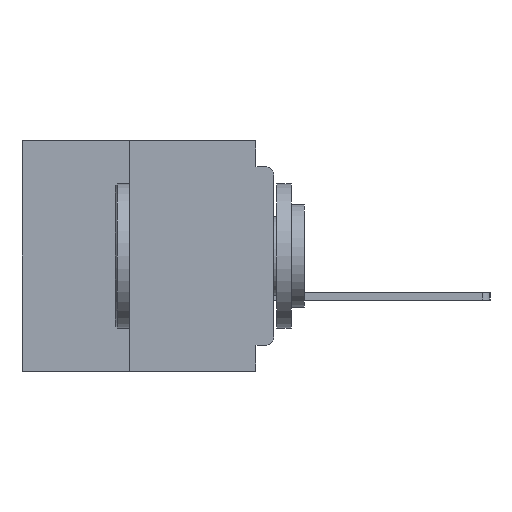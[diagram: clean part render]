
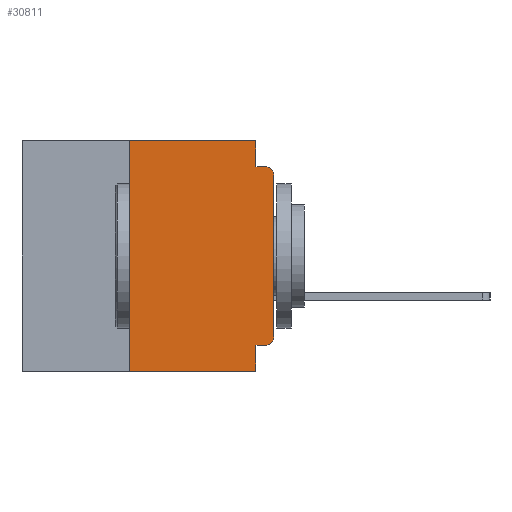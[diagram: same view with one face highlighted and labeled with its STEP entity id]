
A CAD part, left-side view. The second image highlights one B-rep face of the part: STEP entity #30811.
In plain terms, the highlighted planar face has unit normal (-1, 0, 0).
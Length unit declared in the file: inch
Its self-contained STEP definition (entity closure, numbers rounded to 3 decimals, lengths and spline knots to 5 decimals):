
#377 = CARTESIAN_POINT ( 'NONE',  ( 0., 0.031, -0.4 ) ) ;
#477 = LINE ( 'NONE', #377, #32429 ) ;
#690 = ORIENTED_EDGE ( 'NONE', *, *, #26634, .F. ) ;
#1308 = CARTESIAN_POINT ( 'NONE',  ( 0., 0.25, 0. ) ) ;
#2202 = EDGE_CURVE ( 'NONE', #17226, #9035, #2603, .T. ) ;
#2603 = LINE ( 'NONE', #23294, #18097 ) ;
#2668 = DIRECTION ( 'NONE',  ( 0., -1., 0. ) ) ;
#2784 = DIRECTION ( 'NONE',  ( 0., -1., 0. ) ) ;
#3067 = EDGE_CURVE ( 'NONE', #31469, #33344, #477, .T. ) ;
#4075 = ORIENTED_EDGE ( 'NONE', *, *, #11800, .F. ) ;
#4390 = ORIENTED_EDGE ( 'NONE', *, *, #16983, .T. ) ;
#4694 = CIRCLE ( 'NONE', #15350, 0.015 ) ;
#4829 = DIRECTION ( 'NONE',  ( 0., 1., 0. ) ) ;
#4924 = DIRECTION ( 'NONE',  ( -1., 0., 0. ) ) ;
#4970 = VERTEX_POINT ( 'NONE', #20341 ) ;
#5409 = ORIENTED_EDGE ( 'NONE', *, *, #3067, .F. ) ;
#5547 = VECTOR ( 'NONE', #8310, 39.37008 ) ;
#5725 = CARTESIAN_POINT ( 'NONE',  ( 0., 0.437, 0. ) ) ;
#6481 = LINE ( 'NONE', #14185, #12767 ) ;
#6524 = LINE ( 'NONE', #39136, #5547 ) ;
#7048 = CARTESIAN_POINT ( 'NONE',  ( 0., 0.031, 0. ) ) ;
#7213 = LINE ( 'NONE', #18209, #15470 ) ;
#7415 = DIRECTION ( 'NONE',  ( 0., 0., -1. ) ) ;
#8310 = DIRECTION ( 'NONE',  ( 0., 0., 1. ) ) ;
#8860 = DIRECTION ( 'NONE',  ( 0., 0., -1. ) ) ;
#9035 = VERTEX_POINT ( 'NONE', #18896 ) ;
#9562 = CIRCLE ( 'NONE', #22110, 0.015 ) ;
#10268 = CARTESIAN_POINT ( 'NONE',  ( 0., 0.437, -0.4 ) ) ;
#11218 = CARTESIAN_POINT ( 'NONE',  ( 0., 0.015, -0.355 ) ) ;
#11800 = EDGE_CURVE ( 'NONE', #15810, #4970, #7213, .T. ) ;
#12302 = AXIS2_PLACEMENT_3D ( 'NONE', #5725, #27368, #8860 ) ;
#12767 = VECTOR ( 'NONE', #4829, 39.37008 ) ;
#12866 = EDGE_CURVE ( 'NONE', #27410, #9035, #9562, .T. ) ;
#13295 = DIRECTION ( 'NONE',  ( 0., 0., 1. ) ) ;
#14185 = CARTESIAN_POINT ( 'NONE',  ( 0., 0., -0.355 ) ) ;
#14215 = DIRECTION ( 'NONE',  ( -1., 0., 0. ) ) ;
#14972 = VERTEX_POINT ( 'NONE', #39874 ) ;
#15350 = AXIS2_PLACEMENT_3D ( 'NONE', #23416, #4924, #26543 ) ;
#15470 = VECTOR ( 'NONE', #2784, 39.37008 ) ;
#15810 = VERTEX_POINT ( 'NONE', #1308 ) ;
#16983 = EDGE_CURVE ( 'NONE', #14972, #33344, #32360, .T. ) ;
#17226 = VERTEX_POINT ( 'NONE', #17668 ) ;
#17668 = CARTESIAN_POINT ( 'NONE',  ( 0., 0.031, -0.045 ) ) ;
#18097 = VECTOR ( 'NONE', #2668, 39.37008 ) ;
#18209 = CARTESIAN_POINT ( 'NONE',  ( 0., 0.437, 0. ) ) ;
#18896 = CARTESIAN_POINT ( 'NONE',  ( 0., 0.015, -0.045 ) ) ;
#19256 = EDGE_CURVE ( 'NONE', #34540, #27410, #6524, .T. ) ;
#20341 = CARTESIAN_POINT ( 'NONE',  ( 0., 0.031, 0. ) ) ;
#22110 = AXIS2_PLACEMENT_3D ( 'NONE', #32738, #14215, #35847 ) ;
#22524 = EDGE_CURVE ( 'NONE', #23639, #31469, #6481, .T. ) ;
#22664 = DIRECTION ( 'NONE',  ( 0., -1., 0. ) ) ;
#22782 = LINE ( 'NONE', #31707, #31092 ) ;
#23105 = VECTOR ( 'NONE', #22664, 39.37008 ) ;
#23294 = CARTESIAN_POINT ( 'NONE',  ( 0., 0., -0.045 ) ) ;
#23416 = CARTESIAN_POINT ( 'NONE',  ( 0., 0.015, -0.34 ) ) ;
#23639 = VERTEX_POINT ( 'NONE', #11218 ) ;
#24402 = CARTESIAN_POINT ( 'NONE',  ( 0., 0.031, -0.4 ) ) ;
#25649 = FACE_OUTER_BOUND ( 'NONE', #30650, .T. ) ;
#25681 = ORIENTED_EDGE ( 'NONE', *, *, #12866, .T. ) ;
#26115 = ORIENTED_EDGE ( 'NONE', *, *, #2202, .F. ) ;
#26490 = ORIENTED_EDGE ( 'NONE', *, *, #34265, .F. ) ;
#26543 = DIRECTION ( 'NONE',  ( 0., 0., -1. ) ) ;
#26634 = EDGE_CURVE ( 'NONE', #4970, #17226, #36172, .T. ) ;
#26944 = VECTOR ( 'NONE', #31661, 39.37008 ) ;
#27368 = DIRECTION ( 'NONE',  ( 1., 0., 0. ) ) ;
#27410 = VERTEX_POINT ( 'NONE', #38479 ) ;
#27498 = EDGE_CURVE ( 'NONE', #23639, #34540, #4694, .T. ) ;
#27715 = ORIENTED_EDGE ( 'NONE', *, *, #19256, .T. ) ;
#29923 = ORIENTED_EDGE ( 'NONE', *, *, #22524, .F. ) ;
#30346 = PLANE ( 'NONE',  #12302 ) ;
#30650 = EDGE_LOOP ( 'NONE', ( #27715, #25681, #26115, #690, #4075, #26490, #4390, #5409, #29923, #30844 ) ) ;
#30811 = ADVANCED_FACE ( 'NONE', ( #25649 ), #30346, .F. ) ;
#30844 = ORIENTED_EDGE ( 'NONE', *, *, #27498, .T. ) ;
#31092 = VECTOR ( 'NONE', #13295, 39.37008 ) ;
#31469 = VERTEX_POINT ( 'NONE', #33246 ) ;
#31661 = DIRECTION ( 'NONE',  ( 0., 0., -1. ) ) ;
#31707 = CARTESIAN_POINT ( 'NONE',  ( 0., 0.25, -0.4 ) ) ;
#32360 = LINE ( 'NONE', #10268, #23105 ) ;
#32429 = VECTOR ( 'NONE', #7415, 39.37008 ) ;
#32738 = CARTESIAN_POINT ( 'NONE',  ( 0., 0.015, -0.06 ) ) ;
#32851 = CARTESIAN_POINT ( 'NONE',  ( 0., 0., -0.34 ) ) ;
#33246 = CARTESIAN_POINT ( 'NONE',  ( 0., 0.031, -0.355 ) ) ;
#33344 = VERTEX_POINT ( 'NONE', #24402 ) ;
#34265 = EDGE_CURVE ( 'NONE', #14972, #15810, #22782, .T. ) ;
#34540 = VERTEX_POINT ( 'NONE', #32851 ) ;
#35847 = DIRECTION ( 'NONE',  ( 0., 0., -1. ) ) ;
#36172 = LINE ( 'NONE', #7048, #26944 ) ;
#38479 = CARTESIAN_POINT ( 'NONE',  ( 0., 0., -0.06 ) ) ;
#39136 = CARTESIAN_POINT ( 'NONE',  ( 0., 0., 0. ) ) ;
#39874 = CARTESIAN_POINT ( 'NONE',  ( 0., 0.25, -0.4 ) ) ;
